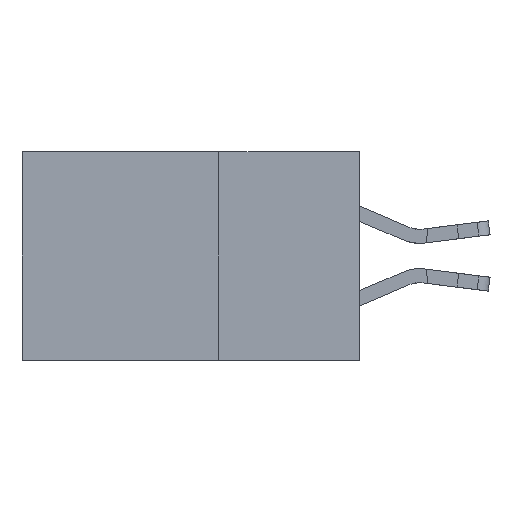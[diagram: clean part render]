
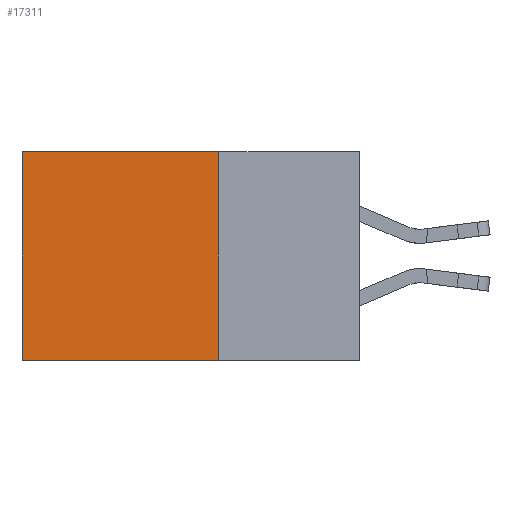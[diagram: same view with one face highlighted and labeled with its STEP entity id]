
A CAD part, left-side view. The second image highlights one B-rep face of the part: STEP entity #17311.
In plain terms, the highlighted planar face has unit normal (-1, 0, 0).
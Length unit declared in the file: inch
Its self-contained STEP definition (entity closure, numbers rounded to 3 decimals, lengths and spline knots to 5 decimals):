
#454 = VERTEX_POINT ( 'NONE', #20147 ) ;
#1841 = ORIENTED_EDGE ( 'NONE', *, *, #31653, .T. ) ;
#2301 = ORIENTED_EDGE ( 'NONE', *, *, #22619, .F. ) ;
#2558 = VERTEX_POINT ( 'NONE', #21853 ) ;
#2736 = FACE_OUTER_BOUND ( 'NONE', #26846, .T. ) ;
#6253 = CARTESIAN_POINT ( 'NONE',  ( 0.2875, 0.25, 0. ) ) ;
#6580 = DIRECTION ( 'NONE',  ( 0., 0., -1. ) ) ;
#8234 = CARTESIAN_POINT ( 'NONE',  ( 0.2875, 0.25, 0. ) ) ;
#8843 = CARTESIAN_POINT ( 'NONE',  ( 0.2875, 0.25, -0.37 ) ) ;
#9283 = VERTEX_POINT ( 'NONE', #29963 ) ;
#9448 = VECTOR ( 'NONE', #14344, 39.37008 ) ;
#9632 = AXIS2_PLACEMENT_3D ( 'NONE', #8234, #11088, #30242 ) ;
#10620 = ORIENTED_EDGE ( 'NONE', *, *, #28009, .F. ) ;
#10660 = VERTEX_POINT ( 'NONE', #8843 ) ;
#10681 = CARTESIAN_POINT ( 'NONE',  ( 0.2875, 0.25, -0.37 ) ) ;
#11088 = DIRECTION ( 'NONE',  ( 1., 0., 0. ) ) ;
#11184 = LINE ( 'NONE', #6253, #17621 ) ;
#13511 = VECTOR ( 'NONE', #6580, 39.37008 ) ;
#14344 = DIRECTION ( 'NONE',  ( 0., 0., -1. ) ) ;
#14923 = CARTESIAN_POINT ( 'NONE',  ( 0.2875, 0.6, 0. ) ) ;
#17311 = ADVANCED_FACE ( 'NONE', ( #2736 ), #27497, .F. ) ;
#17621 = VECTOR ( 'NONE', #22862, 39.37008 ) ;
#20147 = CARTESIAN_POINT ( 'NONE',  ( 0.2875, 0.6, 0. ) ) ;
#20769 = LINE ( 'NONE', #14923, #13511 ) ;
#21853 = CARTESIAN_POINT ( 'NONE',  ( 0.2875, 0.25, 0. ) ) ;
#22619 = EDGE_CURVE ( 'NONE', #2558, #10660, #24088, .T. ) ;
#22862 = DIRECTION ( 'NONE',  ( 0., 1., 0. ) ) ;
#24088 = LINE ( 'NONE', #25227, #9448 ) ;
#25227 = CARTESIAN_POINT ( 'NONE',  ( 0.2875, 0.25, 0. ) ) ;
#26101 = ORIENTED_EDGE ( 'NONE', *, *, #34435, .T. ) ;
#26846 = EDGE_LOOP ( 'NONE', ( #26101, #10620, #2301, #1841 ) ) ;
#27497 = PLANE ( 'NONE',  #9632 ) ;
#28009 = EDGE_CURVE ( 'NONE', #10660, #9283, #29466, .T. ) ;
#28599 = VECTOR ( 'NONE', #35268, 39.37008 ) ;
#29466 = LINE ( 'NONE', #10681, #28599 ) ;
#29963 = CARTESIAN_POINT ( 'NONE',  ( 0.2875, 0.6, -0.37 ) ) ;
#30242 = DIRECTION ( 'NONE',  ( 0., 0., -1. ) ) ;
#31653 = EDGE_CURVE ( 'NONE', #2558, #454, #11184, .T. ) ;
#34435 = EDGE_CURVE ( 'NONE', #454, #9283, #20769, .T. ) ;
#35268 = DIRECTION ( 'NONE',  ( 0., 1., 0. ) ) ;
